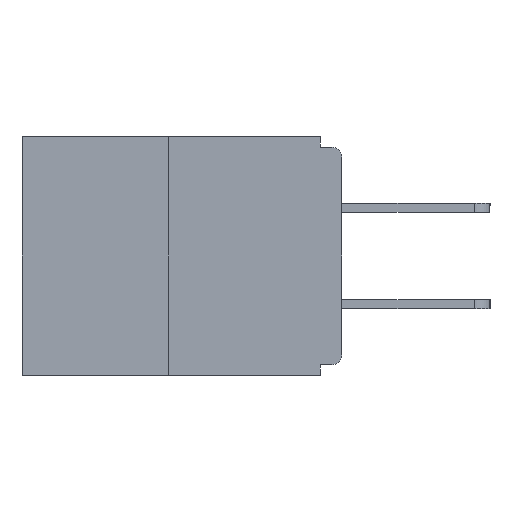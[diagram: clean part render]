
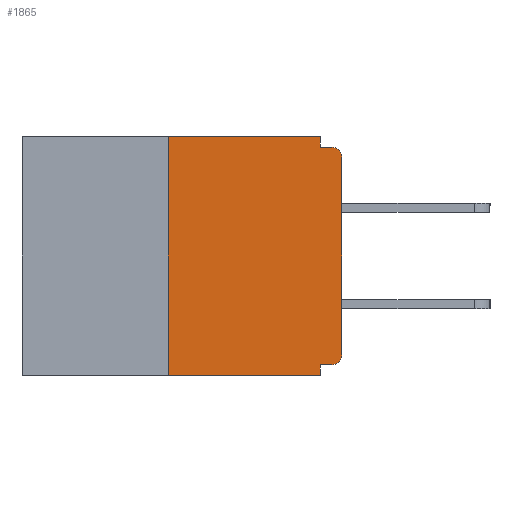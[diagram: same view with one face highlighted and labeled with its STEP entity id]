
A CAD part, left-side view. The second image highlights one B-rep face of the part: STEP entity #1865.
In plain terms, the highlighted planar face has unit normal (-1, 0, 0).
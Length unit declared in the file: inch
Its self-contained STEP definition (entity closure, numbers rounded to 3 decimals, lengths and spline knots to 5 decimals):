
#106 = VECTOR ( 'NONE', #12491, 39.37008 ) ;
#256 = LINE ( 'NONE', #10397, #10120 ) ;
#614 = LINE ( 'NONE', #10161, #2107 ) ;
#653 = VERTEX_POINT ( 'NONE', #1138 ) ;
#719 = VERTEX_POINT ( 'NONE', #18307 ) ;
#955 = ORIENTED_EDGE ( 'NONE', *, *, #7215, .T. ) ;
#1020 = ORIENTED_EDGE ( 'NONE', *, *, #5920, .F. ) ;
#1044 = DIRECTION ( 'NONE',  ( 1., 0., 0. ) ) ;
#1070 = VERTEX_POINT ( 'NONE', #13028 ) ;
#1096 = DIRECTION ( 'NONE',  ( -1., 0., 0. ) ) ;
#1117 = LINE ( 'NONE', #6175, #106 ) ;
#1138 = CARTESIAN_POINT ( 'NONE',  ( 0., 0.031, 0. ) ) ;
#1581 = VECTOR ( 'NONE', #14336, 39.37008 ) ;
#1865 = ADVANCED_FACE ( 'NONE', ( #18388 ), #18281, .F. ) ;
#1947 = EDGE_CURVE ( 'NONE', #1070, #3133, #15869, .T. ) ;
#2107 = VECTOR ( 'NONE', #2316, 39.37008 ) ;
#2151 = CARTESIAN_POINT ( 'NONE',  ( 0., 0., -0.313 ) ) ;
#2306 = CARTESIAN_POINT ( 'NONE',  ( 0., 0.031, 0. ) ) ;
#2316 = DIRECTION ( 'NONE',  ( 0., 1., 0. ) ) ;
#2393 = CARTESIAN_POINT ( 'NONE',  ( 0., 0., -0.03 ) ) ;
#3133 = VERTEX_POINT ( 'NONE', #14000 ) ;
#3661 = DIRECTION ( 'NONE',  ( -1., 0., 0. ) ) ;
#4482 = DIRECTION ( 'NONE',  ( 0., 0., -1. ) ) ;
#5412 = AXIS2_PLACEMENT_3D ( 'NONE', #8890, #1096, #4482 ) ;
#5828 = VERTEX_POINT ( 'NONE', #2151 ) ;
#5920 = EDGE_CURVE ( 'NONE', #18391, #7012, #256, .T. ) ;
#6175 = CARTESIAN_POINT ( 'NONE',  ( 0., 0.46, -0.343 ) ) ;
#6401 = ORIENTED_EDGE ( 'NONE', *, *, #1947, .F. ) ;
#7012 = VERTEX_POINT ( 'NONE', #15163 ) ;
#7215 = EDGE_CURVE ( 'NONE', #5828, #11285, #7248, .T. ) ;
#7248 = LINE ( 'NONE', #16472, #1581 ) ;
#7923 = DIRECTION ( 'NONE',  ( 0., -1., 0. ) ) ;
#8266 = CIRCLE ( 'NONE', #5412, 0.015 ) ;
#8796 = EDGE_LOOP ( 'NONE', ( #16403, #18363, #18165, #1020, #19725, #11465, #955, #12782, #6401, #16415 ) ) ;
#8890 = CARTESIAN_POINT ( 'NONE',  ( 0., 0.015, -0.03 ) ) ;
#8897 = DIRECTION ( 'NONE',  ( 0., 0., -1. ) ) ;
#9388 = CARTESIAN_POINT ( 'NONE',  ( 0., 0.031, -0.328 ) ) ;
#9451 = CARTESIAN_POINT ( 'NONE',  ( 0., 0.25, -0.343 ) ) ;
#9802 = VECTOR ( 'NONE', #20330, 39.37008 ) ;
#10120 = VECTOR ( 'NONE', #8897, 39.37008 ) ;
#10161 = CARTESIAN_POINT ( 'NONE',  ( 0., 0., -0.328 ) ) ;
#10350 = VERTEX_POINT ( 'NONE', #9451 ) ;
#10397 = CARTESIAN_POINT ( 'NONE',  ( 0., 0.031, -0.343 ) ) ;
#11027 = CARTESIAN_POINT ( 'NONE',  ( 0., 0., -0.015 ) ) ;
#11285 = VERTEX_POINT ( 'NONE', #2393 ) ;
#11465 = ORIENTED_EDGE ( 'NONE', *, *, #17586, .T. ) ;
#11605 = DIRECTION ( 'NONE',  ( 0., 0., -1. ) ) ;
#12042 = DIRECTION ( 'NONE',  ( 0., 0., -1. ) ) ;
#12351 = EDGE_CURVE ( 'NONE', #719, #18391, #614, .T. ) ;
#12388 = CARTESIAN_POINT ( 'NONE',  ( 0., 0.46, 0. ) ) ;
#12394 = EDGE_CURVE ( 'NONE', #10350, #7012, #1117, .T. ) ;
#12491 = DIRECTION ( 'NONE',  ( 0., -1., 0. ) ) ;
#12782 = ORIENTED_EDGE ( 'NONE', *, *, #16873, .T. ) ;
#12937 = CARTESIAN_POINT ( 'NONE',  ( 0., 0.25, 0. ) ) ;
#13028 = CARTESIAN_POINT ( 'NONE',  ( 0., 0.031, -0.015 ) ) ;
#13057 = CARTESIAN_POINT ( 'NONE',  ( 0., 0.015, -0.313 ) ) ;
#13933 = AXIS2_PLACEMENT_3D ( 'NONE', #12388, #1044, #12042 ) ;
#14000 = CARTESIAN_POINT ( 'NONE',  ( 0., 0.015, -0.015 ) ) ;
#14119 = LINE ( 'NONE', #16420, #17860 ) ;
#14134 = CARTESIAN_POINT ( 'NONE',  ( 0., 0.46, 0. ) ) ;
#14336 = DIRECTION ( 'NONE',  ( 0., 0., 1. ) ) ;
#14437 = DIRECTION ( 'NONE',  ( 0., 0., -1. ) ) ;
#14497 = EDGE_CURVE ( 'NONE', #653, #1070, #19922, .T. ) ;
#14720 = VECTOR ( 'NONE', #11605, 39.37008 ) ;
#15163 = CARTESIAN_POINT ( 'NONE',  ( 0., 0.031, -0.343 ) ) ;
#15855 = CIRCLE ( 'NONE', #19215, 0.015 ) ;
#15869 = LINE ( 'NONE', #11027, #9802 ) ;
#16266 = LINE ( 'NONE', #14134, #20206 ) ;
#16403 = ORIENTED_EDGE ( 'NONE', *, *, #19132, .F. ) ;
#16415 = ORIENTED_EDGE ( 'NONE', *, *, #14497, .F. ) ;
#16420 = CARTESIAN_POINT ( 'NONE',  ( 0., 0.25, 0. ) ) ;
#16472 = CARTESIAN_POINT ( 'NONE',  ( 0., 0., 0. ) ) ;
#16873 = EDGE_CURVE ( 'NONE', #11285, #3133, #8266, .T. ) ;
#17168 = EDGE_CURVE ( 'NONE', #10350, #19364, #14119, .T. ) ;
#17586 = EDGE_CURVE ( 'NONE', #719, #5828, #15855, .T. ) ;
#17860 = VECTOR ( 'NONE', #19295, 39.37008 ) ;
#18165 = ORIENTED_EDGE ( 'NONE', *, *, #12394, .T. ) ;
#18281 = PLANE ( 'NONE',  #13933 ) ;
#18307 = CARTESIAN_POINT ( 'NONE',  ( 0., 0.015, -0.328 ) ) ;
#18363 = ORIENTED_EDGE ( 'NONE', *, *, #17168, .F. ) ;
#18388 = FACE_OUTER_BOUND ( 'NONE', #8796, .T. ) ;
#18391 = VERTEX_POINT ( 'NONE', #9388 ) ;
#19132 = EDGE_CURVE ( 'NONE', #19364, #653, #16266, .T. ) ;
#19215 = AXIS2_PLACEMENT_3D ( 'NONE', #13057, #3661, #14437 ) ;
#19295 = DIRECTION ( 'NONE',  ( 0., 0., 1. ) ) ;
#19364 = VERTEX_POINT ( 'NONE', #12937 ) ;
#19725 = ORIENTED_EDGE ( 'NONE', *, *, #12351, .F. ) ;
#19922 = LINE ( 'NONE', #2306, #14720 ) ;
#20206 = VECTOR ( 'NONE', #7923, 39.37008 ) ;
#20330 = DIRECTION ( 'NONE',  ( 0., -1., 0. ) ) ;
